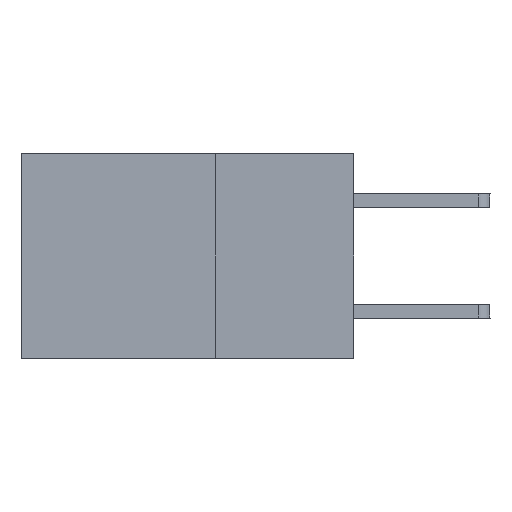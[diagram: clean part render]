
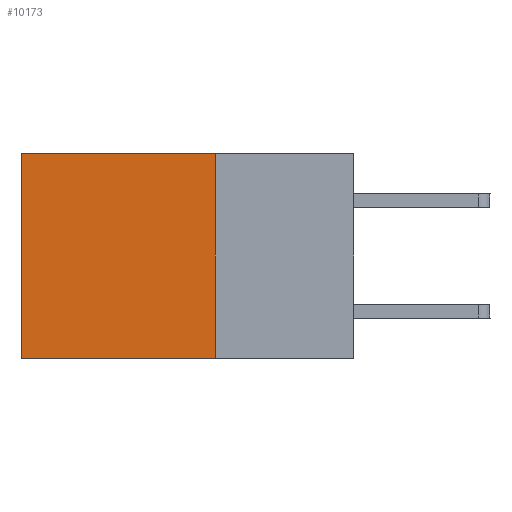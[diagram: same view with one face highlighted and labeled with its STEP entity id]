
A CAD part, left-side view. The second image highlights one B-rep face of the part: STEP entity #10173.
In plain terms, the highlighted planar face has unit normal (-1, 0, 0).
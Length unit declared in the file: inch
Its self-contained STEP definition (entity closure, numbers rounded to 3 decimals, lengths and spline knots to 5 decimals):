
#68 = CARTESIAN_POINT ( 'NONE',  ( 0.2875, 0.6, -0.37 ) ) ;
#114 = EDGE_CURVE ( 'NONE', #6447, #3093, #6766, .T. ) ;
#449 = VECTOR ( 'NONE', #5811, 39.37008 ) ;
#1200 = ORIENTED_EDGE ( 'NONE', *, *, #3618, .T. ) ;
#1847 = ORIENTED_EDGE ( 'NONE', *, *, #3359, .F. ) ;
#2024 = VERTEX_POINT ( 'NONE', #68 ) ;
#2253 = VERTEX_POINT ( 'NONE', #11852 ) ;
#2397 = ORIENTED_EDGE ( 'NONE', *, *, #114, .F. ) ;
#2714 = CARTESIAN_POINT ( 'NONE',  ( 0.2875, 0.25, -0.37 ) ) ;
#3093 = VERTEX_POINT ( 'NONE', #5175 ) ;
#3359 = EDGE_CURVE ( 'NONE', #3093, #2024, #5768, .T. ) ;
#3618 = EDGE_CURVE ( 'NONE', #6447, #2253, #11544, .T. ) ;
#3754 = CARTESIAN_POINT ( 'NONE',  ( 0.2875, 0.6, 0. ) ) ;
#5070 = EDGE_LOOP ( 'NONE', ( #9296, #1847, #2397, #1200 ) ) ;
#5175 = CARTESIAN_POINT ( 'NONE',  ( 0.2875, 0.25, -0.37 ) ) ;
#5768 = LINE ( 'NONE', #2714, #8909 ) ;
#5811 = DIRECTION ( 'NONE',  ( 0., 0., -1. ) ) ;
#6261 = DIRECTION ( 'NONE',  ( 0., 0., -1. ) ) ;
#6447 = VERTEX_POINT ( 'NONE', #8168 ) ;
#6453 = VECTOR ( 'NONE', #12834, 39.37008 ) ;
#6766 = LINE ( 'NONE', #7813, #6453 ) ;
#7055 = DIRECTION ( 'NONE',  ( 1., 0., 0. ) ) ;
#7249 = CARTESIAN_POINT ( 'NONE',  ( 0.2875, 0.25, 0. ) ) ;
#7813 = CARTESIAN_POINT ( 'NONE',  ( 0.2875, 0.25, 0. ) ) ;
#8168 = CARTESIAN_POINT ( 'NONE',  ( 0.2875, 0.25, 0. ) ) ;
#8403 = DIRECTION ( 'NONE',  ( 0., 1., 0. ) ) ;
#8606 = CARTESIAN_POINT ( 'NONE',  ( 0.2875, 0.25, 0. ) ) ;
#8909 = VECTOR ( 'NONE', #9012, 39.37008 ) ;
#8943 = VECTOR ( 'NONE', #8403, 39.37008 ) ;
#9012 = DIRECTION ( 'NONE',  ( 0., 1., 0. ) ) ;
#9296 = ORIENTED_EDGE ( 'NONE', *, *, #12480, .T. ) ;
#10173 = ADVANCED_FACE ( 'NONE', ( #11109 ), #10243, .F. ) ;
#10243 = PLANE ( 'NONE',  #11178 ) ;
#11109 = FACE_OUTER_BOUND ( 'NONE', #5070, .T. ) ;
#11178 = AXIS2_PLACEMENT_3D ( 'NONE', #7249, #7055, #6261 ) ;
#11544 = LINE ( 'NONE', #8606, #8943 ) ;
#11852 = CARTESIAN_POINT ( 'NONE',  ( 0.2875, 0.6, 0. ) ) ;
#12480 = EDGE_CURVE ( 'NONE', #2253, #2024, #12875, .T. ) ;
#12834 = DIRECTION ( 'NONE',  ( 0., 0., -1. ) ) ;
#12875 = LINE ( 'NONE', #3754, #449 ) ;
